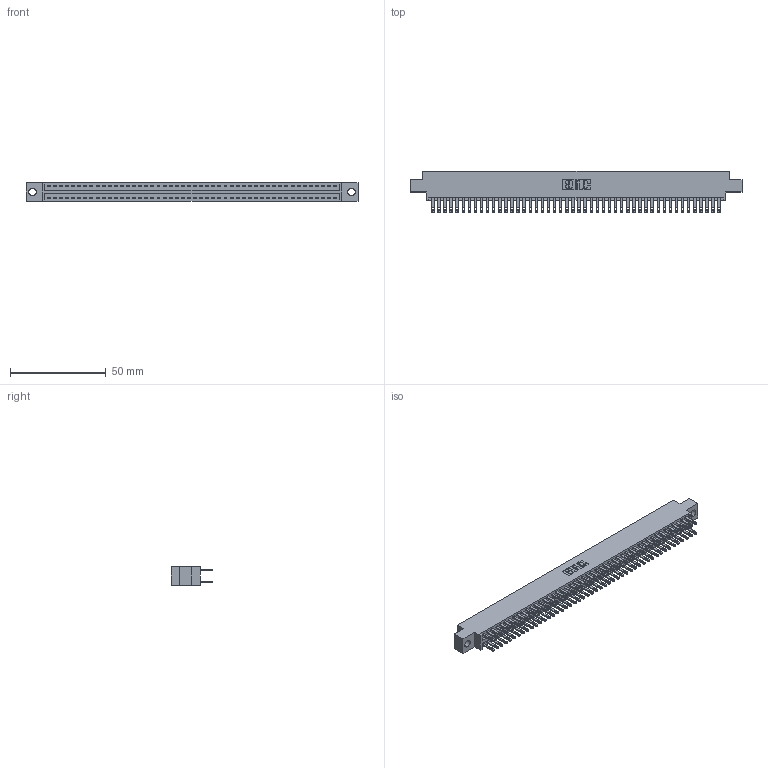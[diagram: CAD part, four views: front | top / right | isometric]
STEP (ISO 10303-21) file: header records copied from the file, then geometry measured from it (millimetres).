
FILE_DESCRIPTION (( 'STEP AP203' ), '1' );
FILE_NAME ('896-096-500-804.STEP', '2021-07-28T03:27:28', ( '' ), ( '' ), 'SwSTEP 2.0', 'SolidWorks 2020', '' );
FILE_SCHEMA (( 'CONFIG_CONTROL_DESIGN' ));
Length unit declared in the file: inch
Products named in the file (3): 846 Part_0.170 Offset - 0.156 Dia-TH; 345-292-001_345-293-100; 896-096-500-804
Assembly tree (97 placements, depth 2):
  896-096-500-804
    846 Part_0.170 Offset - 0.156 Dia-TH
    345-292-001_345-293-100  x96
Bounding box: 172.97 x 21.84 x 9.4 mm (x, y, z)
Volume: 16964.6 mm3; surface area: 24411.1 mm2
Topology: 97 solids, 97 shells, 4734 faces, 14453 edges, 9634 vertices
Faces by surface type: plane 2864, cylinder 1870
Entity records: 30583 total; most frequent: CARTESIAN_POINT 5032, ORIENTED_EDGE 4966, DIRECTION 4487, EDGE_CURVE 2483, VECTOR 2155, LINE 2155, VERTEX_POINT 1654, AXIS2_PLACEMENT_3D 1166
